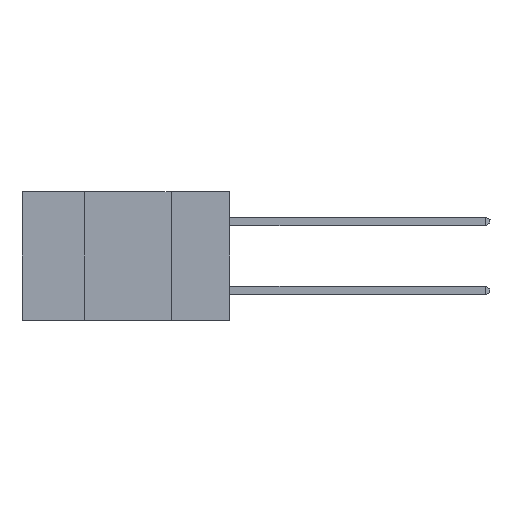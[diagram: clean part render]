
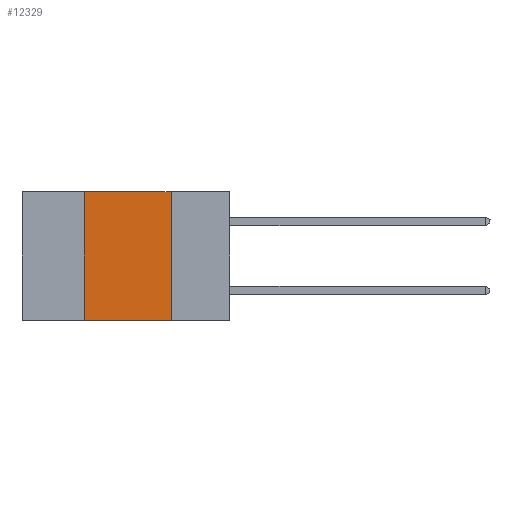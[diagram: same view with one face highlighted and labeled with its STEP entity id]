
A CAD part, left-side view. The second image highlights one B-rep face of the part: STEP entity #12329.
In plain terms, the highlighted planar face has unit normal (-1, 0, 0).
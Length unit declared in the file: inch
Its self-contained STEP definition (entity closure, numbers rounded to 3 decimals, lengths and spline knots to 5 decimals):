
#362 = CARTESIAN_POINT ( 'NONE',  ( 0., 0.42, 0. ) ) ;
#676 = CARTESIAN_POINT ( 'NONE',  ( 0., 0.17, -0.37 ) ) ;
#778 = VERTEX_POINT ( 'NONE', #6013 ) ;
#1571 = LINE ( 'NONE', #676, #2008 ) ;
#1750 = DIRECTION ( 'NONE',  ( 0., 0., 1. ) ) ;
#2008 = VECTOR ( 'NONE', #6055, 39.37008 ) ;
#2171 = CARTESIAN_POINT ( 'NONE',  ( 0., 0.6, 0. ) ) ;
#2441 = EDGE_LOOP ( 'NONE', ( #2836, #12813, #11942, #4371 ) ) ;
#2503 = VERTEX_POINT ( 'NONE', #3114 ) ;
#2688 = DIRECTION ( 'NONE',  ( 1., 0., 0. ) ) ;
#2836 = ORIENTED_EDGE ( 'NONE', *, *, #6313, .F. ) ;
#2965 = CARTESIAN_POINT ( 'NONE',  ( 0., 0.6, 0. ) ) ;
#3044 = EDGE_CURVE ( 'NONE', #5949, #2503, #8209, .T. ) ;
#3114 = CARTESIAN_POINT ( 'NONE',  ( 0., 0.17, -0.37 ) ) ;
#3852 = LINE ( 'NONE', #12163, #10578 ) ;
#4103 = AXIS2_PLACEMENT_3D ( 'NONE', #2965, #2688, #6948 ) ;
#4113 = VERTEX_POINT ( 'NONE', #362 ) ;
#4235 = CARTESIAN_POINT ( 'NONE',  ( 0., 0.42, -0.37 ) ) ;
#4371 = ORIENTED_EDGE ( 'NONE', *, *, #3044, .T. ) ;
#5075 = CARTESIAN_POINT ( 'NONE',  ( 0., 0.6, -0.37 ) ) ;
#5949 = VERTEX_POINT ( 'NONE', #4235 ) ;
#6013 = CARTESIAN_POINT ( 'NONE',  ( 0., 0.17, 0. ) ) ;
#6055 = DIRECTION ( 'NONE',  ( 0., 0., -1. ) ) ;
#6313 = EDGE_CURVE ( 'NONE', #778, #2503, #1571, .T. ) ;
#6948 = DIRECTION ( 'NONE',  ( 0., 0., -1. ) ) ;
#7219 = VECTOR ( 'NONE', #8624, 39.37008 ) ;
#8209 = LINE ( 'NONE', #5075, #13196 ) ;
#8624 = DIRECTION ( 'NONE',  ( 0., -1., 0. ) ) ;
#10569 = DIRECTION ( 'NONE',  ( 0., -1., 0. ) ) ;
#10578 = VECTOR ( 'NONE', #1750, 39.37008 ) ;
#11942 = ORIENTED_EDGE ( 'NONE', *, *, #13350, .F. ) ;
#12163 = CARTESIAN_POINT ( 'NONE',  ( 0., 0.42, -0.37 ) ) ;
#12329 = ADVANCED_FACE ( 'NONE', ( #13455 ), #13595, .F. ) ;
#12447 = EDGE_CURVE ( 'NONE', #4113, #778, #12676, .T. ) ;
#12676 = LINE ( 'NONE', #2171, #7219 ) ;
#12813 = ORIENTED_EDGE ( 'NONE', *, *, #12447, .F. ) ;
#13196 = VECTOR ( 'NONE', #10569, 39.37008 ) ;
#13350 = EDGE_CURVE ( 'NONE', #5949, #4113, #3852, .T. ) ;
#13455 = FACE_OUTER_BOUND ( 'NONE', #2441, .T. ) ;
#13595 = PLANE ( 'NONE',  #4103 ) ;
